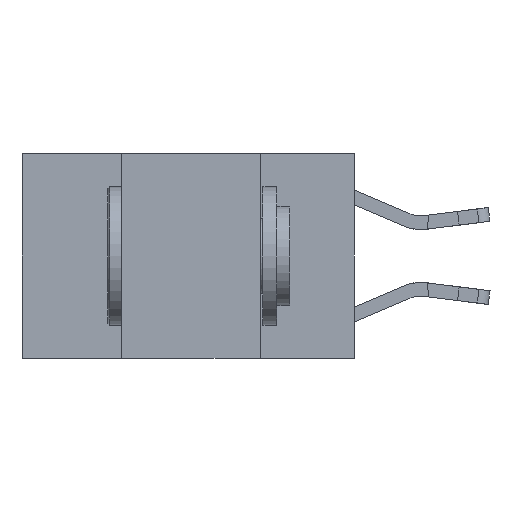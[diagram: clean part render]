
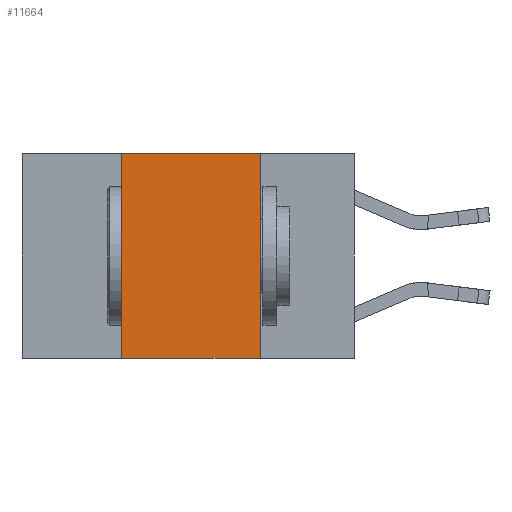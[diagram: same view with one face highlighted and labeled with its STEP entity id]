
A CAD part, left-side view. The second image highlights one B-rep face of the part: STEP entity #11664.
In plain terms, the highlighted planar face has unit normal (-1, 0, 0).
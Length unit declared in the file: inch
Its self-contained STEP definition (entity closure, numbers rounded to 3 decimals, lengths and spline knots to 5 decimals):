
#238 = DIRECTION ( 'NONE',  ( 0., 0., -1. ) ) ;
#241 = VERTEX_POINT ( 'NONE', #16276 ) ;
#410 = EDGE_LOOP ( 'NONE', ( #7012, #10956, #18612, #7480 ) ) ;
#948 = EDGE_CURVE ( 'NONE', #4313, #12819, #16055, .T. ) ;
#4189 = VECTOR ( 'NONE', #238, 39.37008 ) ;
#4288 = FACE_OUTER_BOUND ( 'NONE', #410, .T. ) ;
#4313 = VERTEX_POINT ( 'NONE', #13996 ) ;
#6016 = CARTESIAN_POINT ( 'NONE',  ( 0., 0.42, -0.37 ) ) ;
#6783 = PLANE ( 'NONE',  #6853 ) ;
#6853 = AXIS2_PLACEMENT_3D ( 'NONE', #17011, #8306, #18428 ) ;
#7012 = ORIENTED_EDGE ( 'NONE', *, *, #14380, .F. ) ;
#7480 = ORIENTED_EDGE ( 'NONE', *, *, #17254, .T. ) ;
#7896 = CARTESIAN_POINT ( 'NONE',  ( 0., 0.17, 0. ) ) ;
#8306 = DIRECTION ( 'NONE',  ( 1., 0., 0. ) ) ;
#10927 = CARTESIAN_POINT ( 'NONE',  ( 0., 0.42, 0. ) ) ;
#10956 = ORIENTED_EDGE ( 'NONE', *, *, #948, .F. ) ;
#11217 = VECTOR ( 'NONE', #12401, 39.37008 ) ;
#11664 = ADVANCED_FACE ( 'NONE', ( #4288 ), #6783, .F. ) ;
#12401 = DIRECTION ( 'NONE',  ( 0., 0., 1. ) ) ;
#12819 = VERTEX_POINT ( 'NONE', #19031 ) ;
#13996 = CARTESIAN_POINT ( 'NONE',  ( 0., 0.42, 0. ) ) ;
#14197 = DIRECTION ( 'NONE',  ( 0., -1., 0. ) ) ;
#14380 = EDGE_CURVE ( 'NONE', #12819, #241, #15981, .T. ) ;
#15045 = VECTOR ( 'NONE', #14197, 39.37008 ) ;
#15491 = LINE ( 'NONE', #17141, #15045 ) ;
#15981 = LINE ( 'NONE', #7896, #4189 ) ;
#16055 = LINE ( 'NONE', #17805, #18960 ) ;
#16276 = CARTESIAN_POINT ( 'NONE',  ( 0., 0.17, -0.37 ) ) ;
#16297 = EDGE_CURVE ( 'NONE', #18348, #4313, #18418, .T. ) ;
#17011 = CARTESIAN_POINT ( 'NONE',  ( 0., 0.6, 0. ) ) ;
#17141 = CARTESIAN_POINT ( 'NONE',  ( 0., 0.6, -0.37 ) ) ;
#17254 = EDGE_CURVE ( 'NONE', #18348, #241, #15491, .T. ) ;
#17765 = DIRECTION ( 'NONE',  ( 0., -1., 0. ) ) ;
#17805 = CARTESIAN_POINT ( 'NONE',  ( 0., 0.6, 0. ) ) ;
#18348 = VERTEX_POINT ( 'NONE', #6016 ) ;
#18418 = LINE ( 'NONE', #10927, #11217 ) ;
#18428 = DIRECTION ( 'NONE',  ( 0., 0., -1. ) ) ;
#18612 = ORIENTED_EDGE ( 'NONE', *, *, #16297, .F. ) ;
#18960 = VECTOR ( 'NONE', #17765, 39.37008 ) ;
#19031 = CARTESIAN_POINT ( 'NONE',  ( 0., 0.17, 0. ) ) ;
